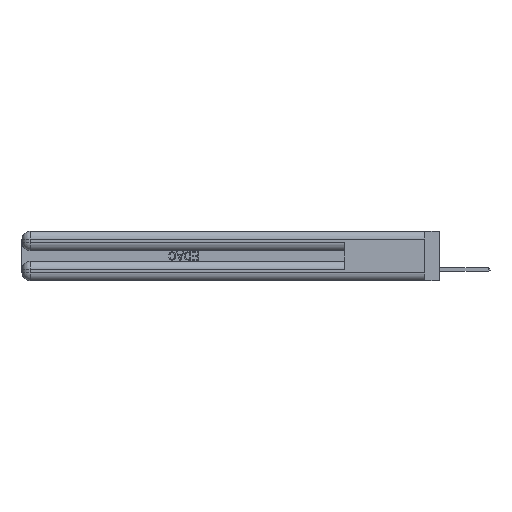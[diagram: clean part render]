
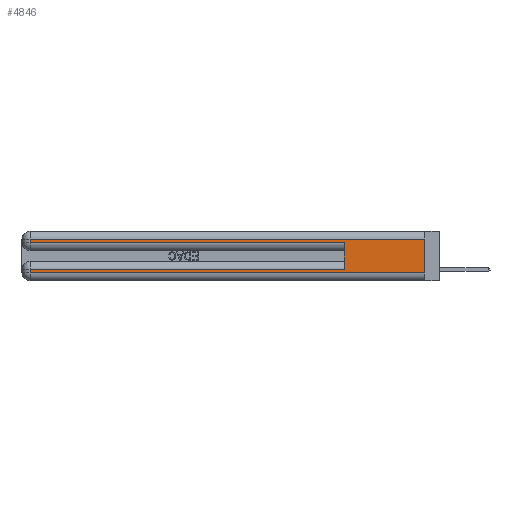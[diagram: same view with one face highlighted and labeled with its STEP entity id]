
A CAD part, left-side view. The second image highlights one B-rep face of the part: STEP entity #4846.
In plain terms, the highlighted planar face has unit normal (-1, 0, 0).
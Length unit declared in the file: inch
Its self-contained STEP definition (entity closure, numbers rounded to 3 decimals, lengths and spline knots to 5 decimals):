
#1131 = CARTESIAN_POINT ( 'NONE',  ( 0., 0., 0.285 ) ) ;
#1515 = DIRECTION ( 'NONE',  ( 0., 0., -1. ) ) ;
#2336 = DIRECTION ( 'NONE',  ( 0., 0., 1. ) ) ;
#3112 = VECTOR ( 'NONE', #2336, 39.37008 ) ;
#3434 = EDGE_CURVE ( 'NONE', #32167, #34531, #54141, .T. ) ;
#3648 = EDGE_CURVE ( 'NONE', #32167, #12823, #29914, .T. ) ;
#4154 = LINE ( 'NONE', #38936, #13908 ) ;
#4846 = ADVANCED_FACE ( 'NONE', ( #41002 ), #19704, .F. ) ;
#10047 = DIRECTION ( 'NONE',  ( 0., -1., 0. ) ) ;
#10703 = CARTESIAN_POINT ( 'NONE',  ( 0., 0., 0.06 ) ) ;
#11701 = CARTESIAN_POINT ( 'NONE',  ( 0., 2.94, 0.285 ) ) ;
#12728 = EDGE_CURVE ( 'NONE', #21340, #12823, #53599, .T. ) ;
#12823 = VERTEX_POINT ( 'NONE', #23701 ) ;
#13908 = VECTOR ( 'NONE', #38769, 39.37008 ) ;
#15373 = ORIENTED_EDGE ( 'NONE', *, *, #17391, .T. ) ;
#15989 = ORIENTED_EDGE ( 'NONE', *, *, #3434, .T. ) ;
#16203 = CARTESIAN_POINT ( 'NONE',  ( 0., 0., 0.31 ) ) ;
#16249 = VECTOR ( 'NONE', #10047, 39.37008 ) ;
#16652 = ORIENTED_EDGE ( 'NONE', *, *, #53275, .T. ) ;
#16715 = DIRECTION ( 'NONE',  ( 0., 1., 0. ) ) ;
#17391 = EDGE_CURVE ( 'NONE', #34531, #38652, #46436, .T. ) ;
#17759 = CARTESIAN_POINT ( 'NONE',  ( 0., 0., 0.06 ) ) ;
#19603 = VECTOR ( 'NONE', #46493, 39.37008 ) ;
#19704 = PLANE ( 'NONE',  #28755 ) ;
#21119 = ORIENTED_EDGE ( 'NONE', *, *, #21175, .T. ) ;
#21175 = EDGE_CURVE ( 'NONE', #38652, #53062, #50691, .T. ) ;
#21340 = VERTEX_POINT ( 'NONE', #11701 ) ;
#22331 = CARTESIAN_POINT ( 'NONE',  ( 0., 2.94, 0.085 ) ) ;
#23362 = ORIENTED_EDGE ( 'NONE', *, *, #3648, .F. ) ;
#23701 = CARTESIAN_POINT ( 'NONE',  ( 0., 0.6, 0.285 ) ) ;
#27144 = DIRECTION ( 'NONE',  ( 1., 0., 0. ) ) ;
#27479 = CARTESIAN_POINT ( 'NONE',  ( 0., 2.94, 0.37 ) ) ;
#28755 = AXIS2_PLACEMENT_3D ( 'NONE', #35210, #27144, #1515 ) ;
#29914 = LINE ( 'NONE', #35671, #3112 ) ;
#30256 = ORIENTED_EDGE ( 'NONE', *, *, #51216, .T. ) ;
#30826 = LINE ( 'NONE', #16203, #33533 ) ;
#31893 = DIRECTION ( 'NONE',  ( 0., 0., -1. ) ) ;
#32167 = VERTEX_POINT ( 'NONE', #39231 ) ;
#33484 = EDGE_CURVE ( 'NONE', #38005, #53062, #4154, .T. ) ;
#33533 = VECTOR ( 'NONE', #16715, 39.37008 ) ;
#34531 = VERTEX_POINT ( 'NONE', #22331 ) ;
#35210 = CARTESIAN_POINT ( 'NONE',  ( 0., 0., 0.37 ) ) ;
#35671 = CARTESIAN_POINT ( 'NONE',  ( 0., 0.6, 0.145 ) ) ;
#36608 = VERTEX_POINT ( 'NONE', #52441 ) ;
#36691 = CARTESIAN_POINT ( 'NONE',  ( 0., 2.94, 0.37 ) ) ;
#38005 = VERTEX_POINT ( 'NONE', #47160 ) ;
#38652 = VERTEX_POINT ( 'NONE', #39831 ) ;
#38769 = DIRECTION ( 'NONE',  ( 0., 0., -1. ) ) ;
#38936 = CARTESIAN_POINT ( 'NONE',  ( 0., 0., 0.37 ) ) ;
#39231 = CARTESIAN_POINT ( 'NONE',  ( 0., 0.6, 0.085 ) ) ;
#39590 = VECTOR ( 'NONE', #52279, 39.37008 ) ;
#39831 = CARTESIAN_POINT ( 'NONE',  ( 0., 2.94, 0.06 ) ) ;
#40152 = ORIENTED_EDGE ( 'NONE', *, *, #12728, .T. ) ;
#40941 = LINE ( 'NONE', #27479, #44829 ) ;
#41002 = FACE_OUTER_BOUND ( 'NONE', #52436, .T. ) ;
#44095 = DIRECTION ( 'NONE',  ( 0., 1., 0. ) ) ;
#44829 = VECTOR ( 'NONE', #31893, 39.37008 ) ;
#46436 = LINE ( 'NONE', #36691, #19603 ) ;
#46493 = DIRECTION ( 'NONE',  ( 0., 0., -1. ) ) ;
#47160 = CARTESIAN_POINT ( 'NONE',  ( 0., 0., 0.31 ) ) ;
#50176 = VECTOR ( 'NONE', #44095, 39.37008 ) ;
#50691 = LINE ( 'NONE', #10703, #39590 ) ;
#51216 = EDGE_CURVE ( 'NONE', #38005, #36608, #30826, .T. ) ;
#52279 = DIRECTION ( 'NONE',  ( 0., -1., 0. ) ) ;
#52436 = EDGE_LOOP ( 'NONE', ( #53631, #30256, #16652, #40152, #23362, #15989, #15373, #21119 ) ) ;
#52441 = CARTESIAN_POINT ( 'NONE',  ( 0., 2.94, 0.31 ) ) ;
#52510 = CARTESIAN_POINT ( 'NONE',  ( 0., 0., 0.085 ) ) ;
#53062 = VERTEX_POINT ( 'NONE', #17759 ) ;
#53275 = EDGE_CURVE ( 'NONE', #36608, #21340, #40941, .T. ) ;
#53599 = LINE ( 'NONE', #1131, #16249 ) ;
#53631 = ORIENTED_EDGE ( 'NONE', *, *, #33484, .F. ) ;
#54141 = LINE ( 'NONE', #52510, #50176 ) ;
